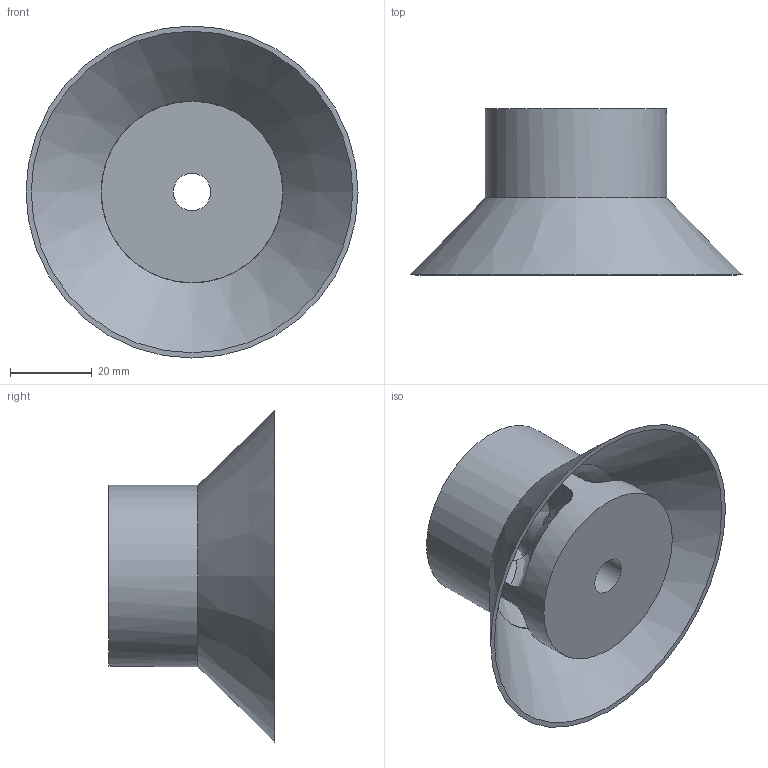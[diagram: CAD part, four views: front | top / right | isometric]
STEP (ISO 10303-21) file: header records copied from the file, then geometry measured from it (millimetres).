
FILE_DESCRIPTION(/* description */ (''),/* implementation_level */ '2;1');
FILE_NAME(/* name */ '1.75 Dia 36 CAL Baffle STEP.step',/* time_stamp */ '2019-05-22T19:20:27-04:00',/* author */ (''),/* organization */ (''),/* preprocessor_version */ 'ST-DEVELOPER v18',/* originating_system */ 'Autodesk Translation Framework v8.2.0.1029',/* authorisation */ '');
FILE_SCHEMA (('AUTOMOTIVE_DESIGN { 1 0 10303 214 3 1 1 }'));
Length unit declared in the file: inch
Products named in the file (1): baf 1.75 dia 1.6 high 36 cal
Bounding box: 81.28 x 40.64 x 81.28 mm (x, y, z)
Volume: 48965.7 mm3; surface area: 23197.4 mm2
Topology: 1 solids, 1 shells, 40 faces, 145 edges, 100 vertices
Faces by surface type: plane 15, bspline 13, cylinder 8, cone 2, torus 2
Full cylindrical faces by diameter (mm): 9.144 x2, 44.45 x2
Entity records: 2291 total; most frequent: CARTESIAN_POINT 1164, ORIENTED_EDGE 290, DIRECTION 158, EDGE_CURVE 145, VERTEX_POINT 100, B_SPLINE_CURVE_WITH_KNOTS 70, AXIS2_PLACEMENT_3D 64, EDGE_LOOP 43
